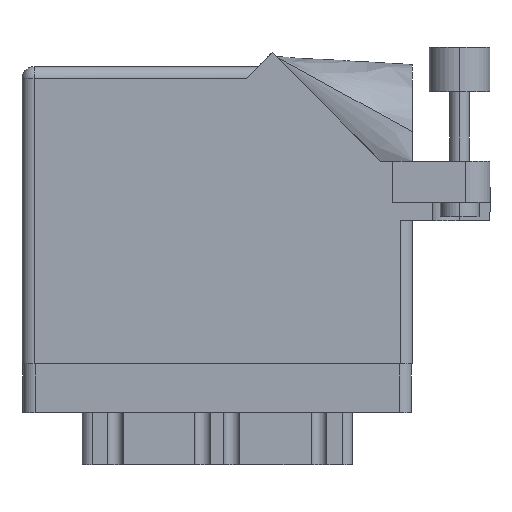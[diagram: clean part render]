
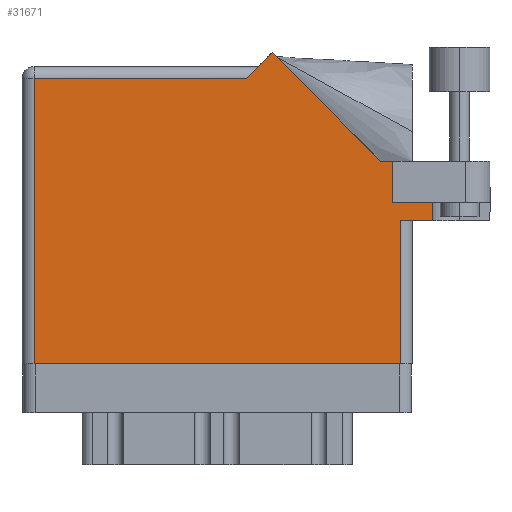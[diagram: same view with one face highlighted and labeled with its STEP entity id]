
A CAD part, front view. The second image highlights one B-rep face of the part: STEP entity #31671.
In plain terms, the highlighted face is planar.
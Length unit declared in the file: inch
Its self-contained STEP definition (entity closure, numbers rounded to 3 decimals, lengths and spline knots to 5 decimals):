
#415 = VECTOR ( 'NONE', #9431, 39.37008 ) ;
#1530 = VERTEX_POINT ( 'NONE', #32522 ) ;
#1922 = VECTOR ( 'NONE', #30445, 39.37008 ) ;
#2114 = CARTESIAN_POINT ( 'NONE',  ( 2.01, 0.737, 0. ) ) ;
#2657 = ORIENTED_EDGE ( 'NONE', *, *, #23064, .F. ) ;
#2682 = EDGE_CURVE ( 'NONE', #31033, #1530, #18324, .T. ) ;
#3004 = ORIENTED_EDGE ( 'NONE', *, *, #9182, .T. ) ;
#3443 = VERTEX_POINT ( 'NONE', #14574 ) ;
#3607 = ORIENTED_EDGE ( 'NONE', *, *, #34518, .T. ) ;
#3886 = LINE ( 'NONE', #11338, #1922 ) ;
#5772 = FACE_OUTER_BOUND ( 'NONE', #27679, .T. ) ;
#5886 = EDGE_CURVE ( 'NONE', #32718, #33464, #32347, .T. ) ;
#5959 = CARTESIAN_POINT ( 'NONE',  ( 2.1115, 0.831, 0. ) ) ;
#6234 = ORIENTED_EDGE ( 'NONE', *, *, #15677, .T. ) ;
#6242 = CARTESIAN_POINT ( 'NONE',  ( 1.84442, 1.044, 0. ) ) ;
#6926 = DIRECTION ( 'NONE',  ( -0.707, -0.707, 0. ) ) ;
#7136 = DIRECTION ( 'NONE',  ( 1., 0., 0. ) ) ;
#7448 = CARTESIAN_POINT ( 'NONE',  ( 1.217, 1.53, 0. ) ) ;
#7474 = CARTESIAN_POINT ( 'NONE',  ( 2.1115, 0.737, 0. ) ) ;
#8110 = CARTESIAN_POINT ( 'NONE',  ( 2.1115, 1.16177, 0. ) ) ;
#9182 = EDGE_CURVE ( 'NONE', #16994, #26439, #3886, .T. ) ;
#9430 = ORIENTED_EDGE ( 'NONE', *, *, #28321, .T. ) ;
#9431 = DIRECTION ( 'NONE',  ( -1., 0., 0. ) ) ;
#9491 = CARTESIAN_POINT ( 'NONE',  ( 1.948, 0.737, 0. ) ) ;
#9620 = AXIS2_PLACEMENT_3D ( 'NONE', #27891, #16556, #14093 ) ;
#9823 = DIRECTION ( 'NONE',  ( 1., 0., 0. ) ) ;
#10090 = LINE ( 'NONE', #2114, #16882 ) ;
#10742 = VECTOR ( 'NONE', #18889, 39.37008 ) ;
#10784 = VECTOR ( 'NONE', #9823, 39.37008 ) ;
#11338 = CARTESIAN_POINT ( 'NONE',  ( 0.062, 0., 0. ) ) ;
#11375 = CARTESIAN_POINT ( 'NONE',  ( 0., 1.468, 0. ) ) ;
#11506 = ORIENTED_EDGE ( 'NONE', *, *, #16292, .T. ) ;
#12001 = VERTEX_POINT ( 'NONE', #18677 ) ;
#12296 = VECTOR ( 'NONE', #17961, 39.37008 ) ;
#12306 = EDGE_CURVE ( 'NONE', #33016, #15457, #20713, .T. ) ;
#12649 = VECTOR ( 'NONE', #7136, 39.37008 ) ;
#13357 = VECTOR ( 'NONE', #17018, 39.37008 ) ;
#13537 = CARTESIAN_POINT ( 'NONE',  ( 1.28771, 1.60071, 0. ) ) ;
#14093 = DIRECTION ( 'NONE',  ( -1., 0., 0. ) ) ;
#14218 = ORIENTED_EDGE ( 'NONE', *, *, #12306, .T. ) ;
#14264 = CARTESIAN_POINT ( 'NONE',  ( 0.062, 1.468, 0. ) ) ;
#14574 = CARTESIAN_POINT ( 'NONE',  ( 1.84442, 1.044, 0. ) ) ;
#14766 = LINE ( 'NONE', #9491, #18949 ) ;
#15051 = CARTESIAN_POINT ( 'NONE',  ( 0.062, 0., 0. ) ) ;
#15457 = VERTEX_POINT ( 'NONE', #34455 ) ;
#15677 = EDGE_CURVE ( 'NONE', #12001, #30630, #14766, .T. ) ;
#16292 = EDGE_CURVE ( 'NONE', #30630, #33464, #10090, .T. ) ;
#16556 = DIRECTION ( 'NONE',  ( 0., 0., -1. ) ) ;
#16882 = VECTOR ( 'NONE', #29536, 39.37008 ) ;
#16994 = VERTEX_POINT ( 'NONE', #14264 ) ;
#17018 = DIRECTION ( 'NONE',  ( -0.707, 0.707, 0. ) ) ;
#17777 = VECTOR ( 'NONE', #26832, 39.37008 ) ;
#17961 = DIRECTION ( 'NONE',  ( -1., 0., 0. ) ) ;
#18324 = LINE ( 'NONE', #26301, #17777 ) ;
#18677 = CARTESIAN_POINT ( 'NONE',  ( 1.948, 0., 0. ) ) ;
#18889 = DIRECTION ( 'NONE',  ( 0., -1., 0. ) ) ;
#18949 = VECTOR ( 'NONE', #22229, 39.37008 ) ;
#19096 = CARTESIAN_POINT ( 'NONE',  ( 1.91, 0.831, 0. ) ) ;
#19499 = LINE ( 'NONE', #11375, #415 ) ;
#19663 = ORIENTED_EDGE ( 'NONE', *, *, #5886, .F. ) ;
#19786 = ORIENTED_EDGE ( 'NONE', *, *, #29152, .T. ) ;
#20057 = LINE ( 'NONE', #34037, #12649 ) ;
#20454 = LINE ( 'NONE', #31421, #12296 ) ;
#20713 = LINE ( 'NONE', #7448, #26766 ) ;
#22229 = DIRECTION ( 'NONE',  ( 0., 1., 0. ) ) ;
#23064 = EDGE_CURVE ( 'NONE', #31033, #32718, #31390, .T. ) ;
#25742 = CARTESIAN_POINT ( 'NONE',  ( 1.91, 0.831, 0. ) ) ;
#26301 = CARTESIAN_POINT ( 'NONE',  ( 1.91, 0.831, 0. ) ) ;
#26439 = VERTEX_POINT ( 'NONE', #15051 ) ;
#26766 = VECTOR ( 'NONE', #6926, 39.37008 ) ;
#26832 = DIRECTION ( 'NONE',  ( 0., 1., 0. ) ) ;
#27550 = PLANE ( 'NONE',  #9620 ) ;
#27679 = EDGE_LOOP ( 'NONE', ( #3607, #6234, #11506, #19663, #2657, #28874, #19786, #9430, #14218, #30321, #3004 ) ) ;
#27891 = CARTESIAN_POINT ( 'NONE',  ( 0., 1.53, 0. ) ) ;
#28321 = EDGE_CURVE ( 'NONE', #3443, #33016, #30476, .T. ) ;
#28874 = ORIENTED_EDGE ( 'NONE', *, *, #2682, .T. ) ;
#29152 = EDGE_CURVE ( 'NONE', #1530, #3443, #20454, .T. ) ;
#29485 = EDGE_CURVE ( 'NONE', #15457, #16994, #19499, .T. ) ;
#29536 = DIRECTION ( 'NONE',  ( 1., 0., 0. ) ) ;
#30321 = ORIENTED_EDGE ( 'NONE', *, *, #29485, .T. ) ;
#30445 = DIRECTION ( 'NONE',  ( 0., -1., 0. ) ) ;
#30476 = LINE ( 'NONE', #6242, #13357 ) ;
#30630 = VERTEX_POINT ( 'NONE', #31944 ) ;
#31033 = VERTEX_POINT ( 'NONE', #19096 ) ;
#31390 = LINE ( 'NONE', #25742, #10784 ) ;
#31421 = CARTESIAN_POINT ( 'NONE',  ( 2.41, 1.044, 0. ) ) ;
#31671 = ADVANCED_FACE ( 'NONE', ( #5772 ), #27550, .F. ) ;
#31944 = CARTESIAN_POINT ( 'NONE',  ( 1.948, 0.737, 0. ) ) ;
#32347 = LINE ( 'NONE', #8110, #10742 ) ;
#32522 = CARTESIAN_POINT ( 'NONE',  ( 1.91, 1.044, 0. ) ) ;
#32718 = VERTEX_POINT ( 'NONE', #5959 ) ;
#33016 = VERTEX_POINT ( 'NONE', #13537 ) ;
#33464 = VERTEX_POINT ( 'NONE', #7474 ) ;
#34037 = CARTESIAN_POINT ( 'NONE',  ( 0., 0., 0. ) ) ;
#34455 = CARTESIAN_POINT ( 'NONE',  ( 1.155, 1.468, 0. ) ) ;
#34518 = EDGE_CURVE ( 'NONE', #26439, #12001, #20057, .T. ) ;
